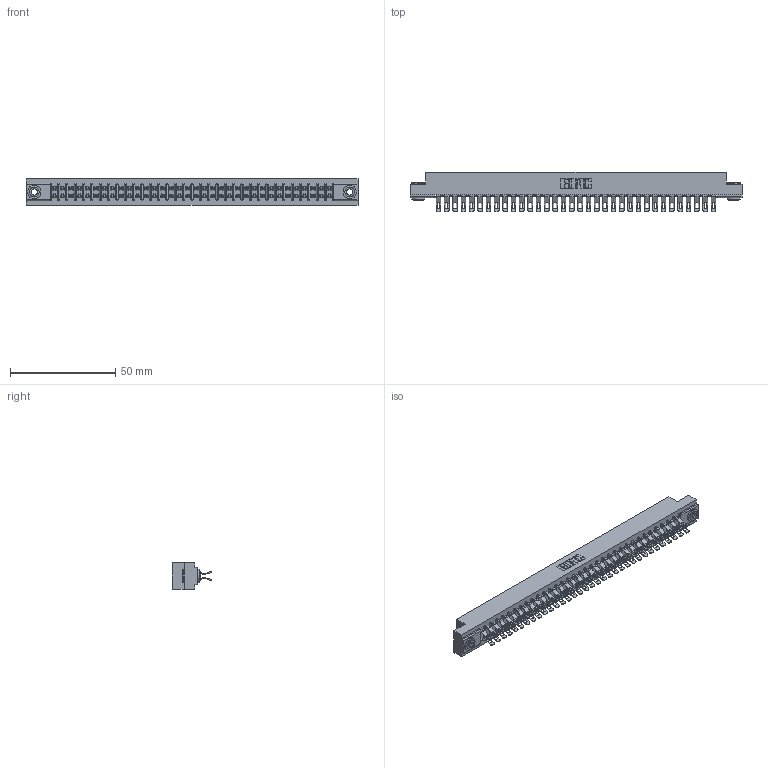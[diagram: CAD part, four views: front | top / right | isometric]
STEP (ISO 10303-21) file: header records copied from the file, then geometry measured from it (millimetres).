
FILE_DESCRIPTION (( 'STEP AP203' ), '1' );
FILE_NAME ('357-068-555-203.STEP', '2018-08-12T18:08:53', ( '' ), ( '' ), 'SwSTEP 2.0', 'SolidWorks 2016', '' );
FILE_SCHEMA (( 'CONFIG_CONTROL_DESIGN' ));
Length unit declared in the file: inch
Products named in the file (4): 345-250-002_345-250-002-102; 357-068-555-203; 307 Part_.156 Dia Mounting Holes; 307-290-001_555
Assembly tree (71 placements, depth 2):
  357-068-555-203
    307 Part_.156 Dia Mounting Holes
    307-290-001_555  x68
    345-250-002_345-250-002-102  x2
Bounding box: 157.73 x 18.75 x 12.7 mm (x, y, z)
Volume: 16920.4 mm3; surface area: 21916.5 mm2
Topology: 71 solids, 71 shells, 4353 faces, 12743 edges, 8306 vertices
Faces by surface type: plane 2406, cylinder 1869, sphere 70, cone 8
Entity records: 32824 total; most frequent: CARTESIAN_POINT 5359, ORIENTED_EDGE 5304, DIRECTION 5274, EDGE_CURVE 2652, VECTOR 2012, LINE 2012, VERTEX_POINT 1716, AXIS2_PLACEMENT_3D 1631
